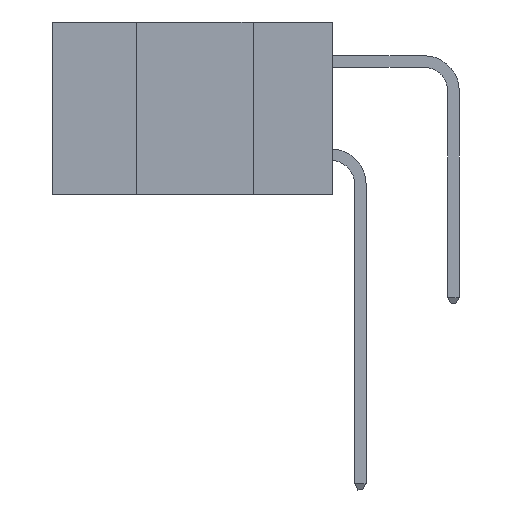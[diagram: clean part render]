
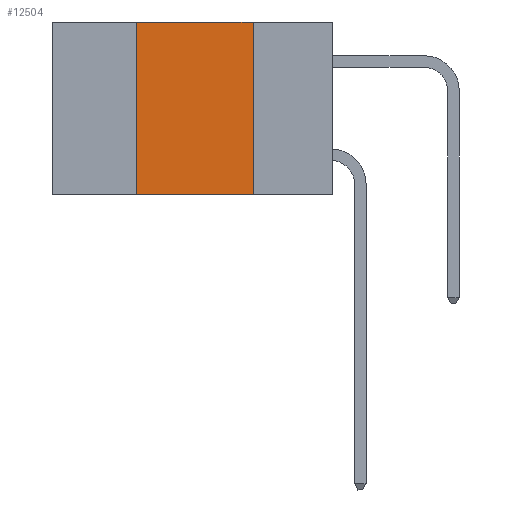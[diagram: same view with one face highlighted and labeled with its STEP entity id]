
A CAD part, left-side view. The second image highlights one B-rep face of the part: STEP entity #12504.
In plain terms, the highlighted planar face has unit normal (-1, 0, 0).
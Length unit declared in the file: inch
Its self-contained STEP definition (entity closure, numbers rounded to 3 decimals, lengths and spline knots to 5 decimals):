
#599 = VERTEX_POINT ( 'NONE', #5453 ) ;
#1070 = DIRECTION ( 'NONE',  ( 0., 0., -1. ) ) ;
#1583 = VERTEX_POINT ( 'NONE', #12095 ) ;
#2036 = ORIENTED_EDGE ( 'NONE', *, *, #4153, .F. ) ;
#3433 = VECTOR ( 'NONE', #11281, 39.37008 ) ;
#4153 = EDGE_CURVE ( 'NONE', #21232, #599, #4296, .T. ) ;
#4296 = LINE ( 'NONE', #22773, #8799 ) ;
#4487 = ORIENTED_EDGE ( 'NONE', *, *, #22190, .F. ) ;
#5453 = CARTESIAN_POINT ( 'NONE',  ( 0., 0.17, 0. ) ) ;
#6250 = VECTOR ( 'NONE', #16793, 39.37008 ) ;
#6458 = CARTESIAN_POINT ( 'NONE',  ( 0., 0.42, -0.37 ) ) ;
#6842 = PLANE ( 'NONE',  #23793 ) ;
#7358 = CARTESIAN_POINT ( 'NONE',  ( 0., 0.17, -0.37 ) ) ;
#8799 = VECTOR ( 'NONE', #9798, 39.37008 ) ;
#9230 = DIRECTION ( 'NONE',  ( 0., 0., -1. ) ) ;
#9798 = DIRECTION ( 'NONE',  ( 0., -1., 0. ) ) ;
#9851 = ORIENTED_EDGE ( 'NONE', *, *, #14787, .F. ) ;
#10538 = EDGE_CURVE ( 'NONE', #17088, #1583, #10671, .T. ) ;
#10671 = LINE ( 'NONE', #14927, #6250 ) ;
#11281 = DIRECTION ( 'NONE',  ( 0., 0., 1. ) ) ;
#12095 = CARTESIAN_POINT ( 'NONE',  ( 0., 0.17, -0.37 ) ) ;
#12481 = DIRECTION ( 'NONE',  ( 1., 0., 0. ) ) ;
#12504 = ADVANCED_FACE ( 'NONE', ( #18339 ), #6842, .F. ) ;
#12986 = VECTOR ( 'NONE', #9230, 39.37008 ) ;
#14787 = EDGE_CURVE ( 'NONE', #599, #1583, #23985, .T. ) ;
#14927 = CARTESIAN_POINT ( 'NONE',  ( 0., 0.6, -0.37 ) ) ;
#14973 = CARTESIAN_POINT ( 'NONE',  ( 0., 0.42, -0.37 ) ) ;
#15881 = CARTESIAN_POINT ( 'NONE',  ( 0., 0.42, 0. ) ) ;
#16633 = EDGE_LOOP ( 'NONE', ( #9851, #2036, #4487, #22617 ) ) ;
#16793 = DIRECTION ( 'NONE',  ( 0., -1., 0. ) ) ;
#17088 = VERTEX_POINT ( 'NONE', #6458 ) ;
#18339 = FACE_OUTER_BOUND ( 'NONE', #16633, .T. ) ;
#21232 = VERTEX_POINT ( 'NONE', #15881 ) ;
#22190 = EDGE_CURVE ( 'NONE', #17088, #21232, #23939, .T. ) ;
#22617 = ORIENTED_EDGE ( 'NONE', *, *, #10538, .T. ) ;
#22773 = CARTESIAN_POINT ( 'NONE',  ( 0., 0.6, 0. ) ) ;
#23586 = CARTESIAN_POINT ( 'NONE',  ( 0., 0.6, 0. ) ) ;
#23793 = AXIS2_PLACEMENT_3D ( 'NONE', #23586, #12481, #1070 ) ;
#23939 = LINE ( 'NONE', #14973, #3433 ) ;
#23985 = LINE ( 'NONE', #7358, #12986 ) ;
